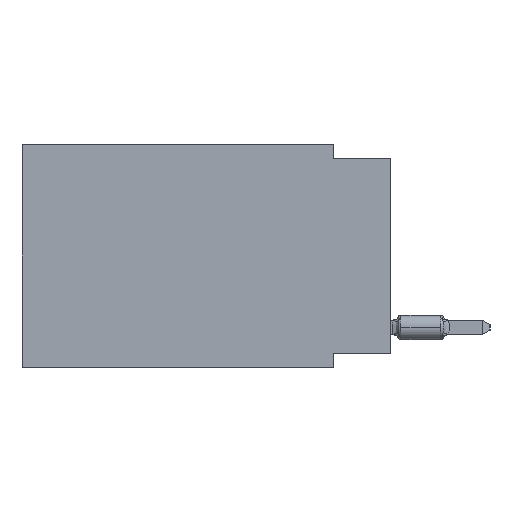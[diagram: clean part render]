
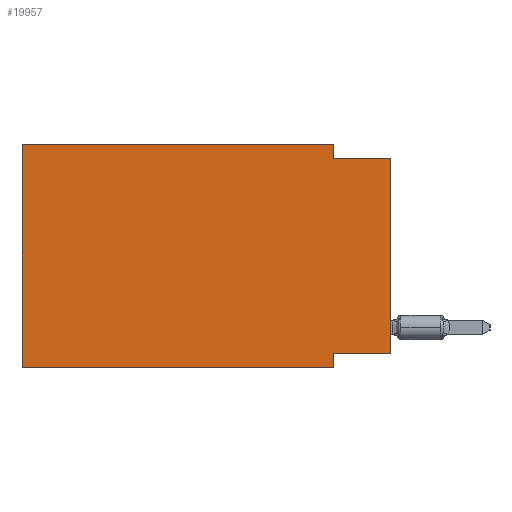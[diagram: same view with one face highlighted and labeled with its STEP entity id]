
A CAD part, left-side view. The second image highlights one B-rep face of the part: STEP entity #19957.
In plain terms, the highlighted planar face has unit normal (-1, 0, 0).
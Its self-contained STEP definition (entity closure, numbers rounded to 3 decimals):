
#80 = CARTESIAN_POINT ( 'NONE',  ( 0., 16.383, 0. ) ) ;
#865 = EDGE_CURVE ( 'NONE', #17270, #13694, #9288, .T. ) ;
#923 = CARTESIAN_POINT ( 'NONE',  ( 0., 0., -0.635 ) ) ;
#1071 = VECTOR ( 'NONE', #13355, 1000. ) ;
#1318 = CARTESIAN_POINT ( 'NONE',  ( 0., 0., -9.271 ) ) ;
#1849 = DIRECTION ( 'NONE',  ( 0., 0., 1. ) ) ;
#1963 = DIRECTION ( 'NONE',  ( 0., 0., -1. ) ) ;
#2086 = FACE_OUTER_BOUND ( 'NONE', #11631, .T. ) ;
#2283 = CARTESIAN_POINT ( 'NONE',  ( 0., 0., -0.635 ) ) ;
#3258 = ORIENTED_EDGE ( 'NONE', *, *, #12839, .F. ) ;
#3988 = CARTESIAN_POINT ( 'NONE',  ( 0., 2.54, -9.271 ) ) ;
#4126 = CARTESIAN_POINT ( 'NONE',  ( 0., 16.383, 0. ) ) ;
#4454 = CARTESIAN_POINT ( 'NONE',  ( 0., 2.54, -9.906 ) ) ;
#5347 = CARTESIAN_POINT ( 'NONE',  ( 0., 16.383, 0. ) ) ;
#5405 = VERTEX_POINT ( 'NONE', #19489 ) ;
#5824 = EDGE_CURVE ( 'NONE', #6891, #5405, #13144, .T. ) ;
#5842 = DIRECTION ( 'NONE',  ( 1., 0., 0. ) ) ;
#6091 = DIRECTION ( 'NONE',  ( 0., 0., -1. ) ) ;
#6549 = VECTOR ( 'NONE', #1849, 1000. ) ;
#6891 = VERTEX_POINT ( 'NONE', #5347 ) ;
#6984 = ORIENTED_EDGE ( 'NONE', *, *, #9974, .F. ) ;
#7007 = ORIENTED_EDGE ( 'NONE', *, *, #16482, .F. ) ;
#7837 = DIRECTION ( 'NONE',  ( 0., -1., 0. ) ) ;
#8637 = EDGE_CURVE ( 'NONE', #17270, #6891, #9233, .T. ) ;
#8888 = VERTEX_POINT ( 'NONE', #923 ) ;
#9233 = LINE ( 'NONE', #80, #10632 ) ;
#9288 = LINE ( 'NONE', #20117, #21720 ) ;
#9638 = LINE ( 'NONE', #2283, #13968 ) ;
#9974 = EDGE_CURVE ( 'NONE', #23098, #13972, #12988, .T. ) ;
#10632 = VECTOR ( 'NONE', #14276, 1000. ) ;
#11134 = ORIENTED_EDGE ( 'NONE', *, *, #865, .T. ) ;
#11631 = EDGE_LOOP ( 'NONE', ( #21020, #7007, #3258, #20723, #20225, #11134, #11646, #6984 ) ) ;
#11646 = ORIENTED_EDGE ( 'NONE', *, *, #19570, .F. ) ;
#12839 = EDGE_CURVE ( 'NONE', #5405, #21131, #22534, .T. ) ;
#12988 = LINE ( 'NONE', #18270, #1071 ) ;
#13064 = CARTESIAN_POINT ( 'NONE',  ( 0., 2.54, -9.906 ) ) ;
#13144 = LINE ( 'NONE', #4126, #21658 ) ;
#13355 = DIRECTION ( 'NONE',  ( 0., 1., 0. ) ) ;
#13540 = AXIS2_PLACEMENT_3D ( 'NONE', #14600, #5842, #1963 ) ;
#13694 = VERTEX_POINT ( 'NONE', #4454 ) ;
#13968 = VECTOR ( 'NONE', #7837, 1000. ) ;
#13972 = VERTEX_POINT ( 'NONE', #3988 ) ;
#14276 = DIRECTION ( 'NONE',  ( 0., 0., 1. ) ) ;
#14600 = CARTESIAN_POINT ( 'NONE',  ( 0., 16.383, 0. ) ) ;
#14697 = DIRECTION ( 'NONE',  ( 0., -1., 0. ) ) ;
#15067 = VECTOR ( 'NONE', #22195, 1000. ) ;
#15211 = LINE ( 'NONE', #18694, #6549 ) ;
#15709 = VECTOR ( 'NONE', #6091, 1000. ) ;
#16482 = EDGE_CURVE ( 'NONE', #21131, #8888, #9638, .T. ) ;
#16909 = LINE ( 'NONE', #13064, #15067 ) ;
#17270 = VERTEX_POINT ( 'NONE', #18220 ) ;
#18220 = CARTESIAN_POINT ( 'NONE',  ( 0., 16.383, -9.906 ) ) ;
#18270 = CARTESIAN_POINT ( 'NONE',  ( 0., 0., -9.271 ) ) ;
#18456 = CARTESIAN_POINT ( 'NONE',  ( 0., 2.54, -0.635 ) ) ;
#18694 = CARTESIAN_POINT ( 'NONE',  ( 0., 0., 0. ) ) ;
#18806 = PLANE ( 'NONE',  #13540 ) ;
#18906 = DIRECTION ( 'NONE',  ( 0., -1., 0. ) ) ;
#19489 = CARTESIAN_POINT ( 'NONE',  ( 0., 2.54, 0. ) ) ;
#19570 = EDGE_CURVE ( 'NONE', #13972, #13694, #16909, .T. ) ;
#19957 = ADVANCED_FACE ( 'NONE', ( #2086 ), #18806, .F. ) ;
#20117 = CARTESIAN_POINT ( 'NONE',  ( 0., 16.383, -9.906 ) ) ;
#20225 = ORIENTED_EDGE ( 'NONE', *, *, #8637, .F. ) ;
#20723 = ORIENTED_EDGE ( 'NONE', *, *, #5824, .F. ) ;
#21020 = ORIENTED_EDGE ( 'NONE', *, *, #21214, .T. ) ;
#21131 = VERTEX_POINT ( 'NONE', #18456 ) ;
#21214 = EDGE_CURVE ( 'NONE', #23098, #8888, #15211, .T. ) ;
#21658 = VECTOR ( 'NONE', #18906, 1000. ) ;
#21720 = VECTOR ( 'NONE', #14697, 1000. ) ;
#22195 = DIRECTION ( 'NONE',  ( 0., 0., -1. ) ) ;
#22534 = LINE ( 'NONE', #22771, #15709 ) ;
#22771 = CARTESIAN_POINT ( 'NONE',  ( 0., 2.54, 0. ) ) ;
#23098 = VERTEX_POINT ( 'NONE', #1318 ) ;
